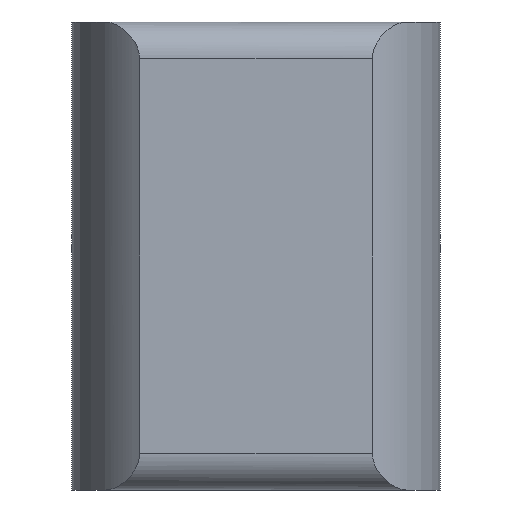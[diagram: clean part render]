
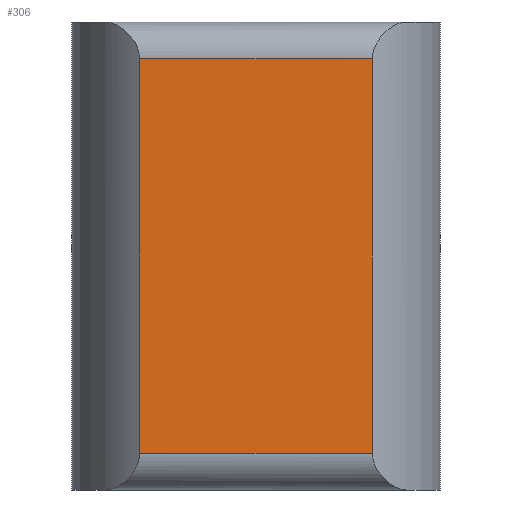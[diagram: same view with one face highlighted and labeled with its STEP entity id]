
A CAD part, left-side view. The second image highlights one B-rep face of the part: STEP entity #306.
In plain terms, the highlighted planar face has unit normal (-1, 0, 0).
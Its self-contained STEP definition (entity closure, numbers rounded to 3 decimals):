
#13 = CARTESIAN_POINT ( 'NONE',  ( -3.875, -3.16, 12.7 ) ) ;
#74 = PLANE ( 'NONE',  #536 ) ;
#76 = VERTEX_POINT ( 'NONE', #389 ) ;
#90 = LINE ( 'NONE', #13, #506 ) ;
#105 = EDGE_CURVE ( 'NONE', #618, #76, #270, .T. ) ;
#111 = VERTEX_POINT ( 'NONE', #492 ) ;
#121 = CARTESIAN_POINT ( 'NONE',  ( -3.875, -3.16, 12.7 ) ) ;
#155 = DIRECTION ( 'NONE',  ( 0., 1., 0. ) ) ;
#195 = EDGE_LOOP ( 'NONE', ( #630, #652, #399, #662 ) ) ;
#270 = LINE ( 'NONE', #661, #597 ) ;
#299 = DIRECTION ( 'NONE',  ( 0., 0., -1. ) ) ;
#306 = ADVANCED_FACE ( 'NONE', ( #392 ), #74, .F. ) ;
#329 = VERTEX_POINT ( 'NONE', #696 ) ;
#354 = LINE ( 'NONE', #481, #430 ) ;
#365 = DIRECTION ( 'NONE',  ( 0., 0., -1. ) ) ;
#377 = VECTOR ( 'NONE', #715, 1000. ) ;
#389 = CARTESIAN_POINT ( 'NONE',  ( -3.875, 3.16, 11.7 ) ) ;
#392 = FACE_OUTER_BOUND ( 'NONE', #195, .T. ) ;
#399 = ORIENTED_EDGE ( 'NONE', *, *, #406, .F. ) ;
#406 = EDGE_CURVE ( 'NONE', #618, #329, #90, .T. ) ;
#424 = DIRECTION ( 'NONE',  ( 0., 1., 0. ) ) ;
#430 = VECTOR ( 'NONE', #365, 1000. ) ;
#476 = DIRECTION ( 'NONE',  ( 1., 0., 0. ) ) ;
#481 = CARTESIAN_POINT ( 'NONE',  ( -3.875, 3.16, 12.7 ) ) ;
#492 = CARTESIAN_POINT ( 'NONE',  ( -3.875, 3.16, 1. ) ) ;
#506 = VECTOR ( 'NONE', #299, 1000. ) ;
#519 = LINE ( 'NONE', #539, #377 ) ;
#536 = AXIS2_PLACEMENT_3D ( 'NONE', #121, #476, #424 ) ;
#539 = CARTESIAN_POINT ( 'NONE',  ( -3.875, -3.16, 1. ) ) ;
#590 = CARTESIAN_POINT ( 'NONE',  ( -3.875, -3.16, 11.7 ) ) ;
#597 = VECTOR ( 'NONE', #155, 1000. ) ;
#604 = EDGE_CURVE ( 'NONE', #111, #329, #519, .T. ) ;
#618 = VERTEX_POINT ( 'NONE', #590 ) ;
#630 = ORIENTED_EDGE ( 'NONE', *, *, #670, .T. ) ;
#652 = ORIENTED_EDGE ( 'NONE', *, *, #604, .T. ) ;
#661 = CARTESIAN_POINT ( 'NONE',  ( -3.875, 3.16, 11.7 ) ) ;
#662 = ORIENTED_EDGE ( 'NONE', *, *, #105, .T. ) ;
#670 = EDGE_CURVE ( 'NONE', #76, #111, #354, .T. ) ;
#696 = CARTESIAN_POINT ( 'NONE',  ( -3.875, -3.16, 1. ) ) ;
#715 = DIRECTION ( 'NONE',  ( 0., -1., 0. ) ) ;
